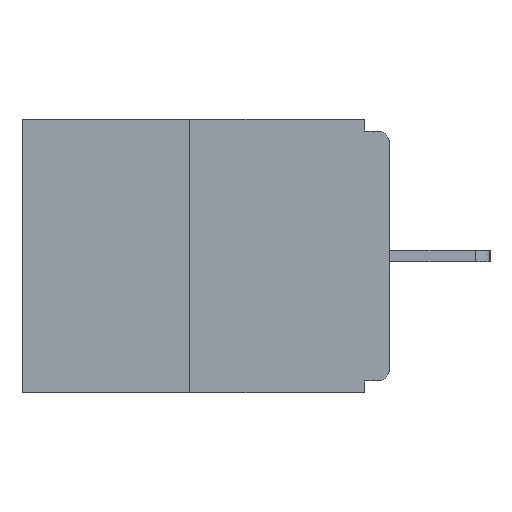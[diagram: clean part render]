
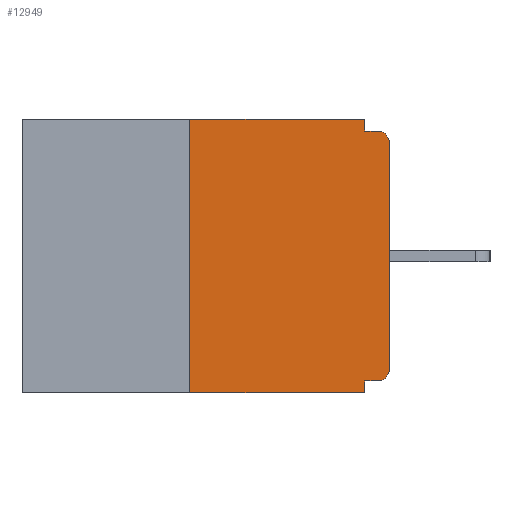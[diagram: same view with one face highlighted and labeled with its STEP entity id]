
A CAD part, left-side view. The second image highlights one B-rep face of the part: STEP entity #12949.
In plain terms, the highlighted planar face has unit normal (-1, 0, 0).
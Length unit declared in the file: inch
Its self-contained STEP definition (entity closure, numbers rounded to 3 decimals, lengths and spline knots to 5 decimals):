
#451 = ORIENTED_EDGE ( 'NONE', *, *, #3247, .T. ) ;
#538 = VERTEX_POINT ( 'NONE', #2615 ) ;
#864 = EDGE_CURVE ( 'NONE', #14884, #14288, #8398, .T. ) ;
#1277 = DIRECTION ( 'NONE',  ( 0., -1., 0. ) ) ;
#1319 = EDGE_CURVE ( 'NONE', #538, #14288, #9498, .T. ) ;
#2554 = PLANE ( 'NONE',  #6915 ) ;
#2615 = CARTESIAN_POINT ( 'NONE',  ( 0., 0.031, -0.015 ) ) ;
#2713 = EDGE_CURVE ( 'NONE', #12094, #3547, #5743, .T. ) ;
#3247 = EDGE_CURVE ( 'NONE', #9905, #14884, #15574, .T. ) ;
#3251 = VERTEX_POINT ( 'NONE', #15971 ) ;
#3293 = CARTESIAN_POINT ( 'NONE',  ( 0., 0.031, 0. ) ) ;
#3547 = VERTEX_POINT ( 'NONE', #12677 ) ;
#3567 = ORIENTED_EDGE ( 'NONE', *, *, #11888, .F. ) ;
#3789 = FACE_OUTER_BOUND ( 'NONE', #4753, .T. ) ;
#4266 = ORIENTED_EDGE ( 'NONE', *, *, #2713, .F. ) ;
#4335 = DIRECTION ( 'NONE',  ( 0., 0., 1. ) ) ;
#4632 = DIRECTION ( 'NONE',  ( 0., -1., 0. ) ) ;
#4753 = EDGE_LOOP ( 'NONE', ( #9517, #4266, #13610, #5436, #12187, #16011, #451, #15184, #11921, #3567 ) ) ;
#4779 = DIRECTION ( 'NONE',  ( 0., 1., 0. ) ) ;
#5211 = CARTESIAN_POINT ( 'NONE',  ( 0., 0.015, -0.328 ) ) ;
#5270 = VECTOR ( 'NONE', #14427, 39.37008 ) ;
#5340 = LINE ( 'NONE', #10348, #9208 ) ;
#5436 = ORIENTED_EDGE ( 'NONE', *, *, #7904, .F. ) ;
#5743 = LINE ( 'NONE', #9524, #14557 ) ;
#6101 = AXIS2_PLACEMENT_3D ( 'NONE', #10490, #6330, #6714 ) ;
#6148 = LINE ( 'NONE', #16160, #8930 ) ;
#6330 = DIRECTION ( 'NONE',  ( -1., 0., 0. ) ) ;
#6335 = DIRECTION ( 'NONE',  ( 0., 0., -1. ) ) ;
#6344 = EDGE_CURVE ( 'NONE', #3547, #9512, #6148, .T. ) ;
#6607 = VECTOR ( 'NONE', #4779, 39.37008 ) ;
#6714 = DIRECTION ( 'NONE',  ( 0., 0., -1. ) ) ;
#6915 = AXIS2_PLACEMENT_3D ( 'NONE', #12328, #7566, #6335 ) ;
#7176 = LINE ( 'NONE', #8628, #6607 ) ;
#7566 = DIRECTION ( 'NONE',  ( 1., 0., 0. ) ) ;
#7615 = AXIS2_PLACEMENT_3D ( 'NONE', #15914, #12053, #13526 ) ;
#7760 = EDGE_CURVE ( 'NONE', #8269, #9905, #13180, .T. ) ;
#7904 = EDGE_CURVE ( 'NONE', #3251, #12931, #8270, .T. ) ;
#8196 = CARTESIAN_POINT ( 'NONE',  ( 0., 0.031, -0.343 ) ) ;
#8269 = VERTEX_POINT ( 'NONE', #5211 ) ;
#8270 = LINE ( 'NONE', #8196, #5270 ) ;
#8398 = CIRCLE ( 'NONE', #7615, 0.015 ) ;
#8628 = CARTESIAN_POINT ( 'NONE',  ( 0., 0., -0.328 ) ) ;
#8690 = CARTESIAN_POINT ( 'NONE',  ( 0., 0.25, -0.343 ) ) ;
#8851 = EDGE_CURVE ( 'NONE', #8269, #3251, #7176, .T. ) ;
#8930 = VECTOR ( 'NONE', #1277, 39.37008 ) ;
#9208 = VECTOR ( 'NONE', #15346, 39.37008 ) ;
#9333 = DIRECTION ( 'NONE',  ( 0., 0., 1. ) ) ;
#9445 = DIRECTION ( 'NONE',  ( 0., 0., -1. ) ) ;
#9498 = LINE ( 'NONE', #15888, #11288 ) ;
#9512 = VERTEX_POINT ( 'NONE', #13851 ) ;
#9517 = ORIENTED_EDGE ( 'NONE', *, *, #6344, .F. ) ;
#9524 = CARTESIAN_POINT ( 'NONE',  ( 0., 0.25, 0. ) ) ;
#9643 = VECTOR ( 'NONE', #9333, 39.37008 ) ;
#9905 = VERTEX_POINT ( 'NONE', #12747 ) ;
#9947 = CARTESIAN_POINT ( 'NONE',  ( 0., 0., -0.03 ) ) ;
#10348 = CARTESIAN_POINT ( 'NONE',  ( 0., 0.46, -0.343 ) ) ;
#10490 = CARTESIAN_POINT ( 'NONE',  ( 0., 0.015, -0.313 ) ) ;
#10599 = EDGE_CURVE ( 'NONE', #12094, #12931, #5340, .T. ) ;
#11288 = VECTOR ( 'NONE', #4632, 39.37008 ) ;
#11347 = CARTESIAN_POINT ( 'NONE',  ( 0., 0.031, -0.343 ) ) ;
#11888 = EDGE_CURVE ( 'NONE', #9512, #538, #13299, .T. ) ;
#11921 = ORIENTED_EDGE ( 'NONE', *, *, #1319, .F. ) ;
#12053 = DIRECTION ( 'NONE',  ( -1., 0., 0. ) ) ;
#12094 = VERTEX_POINT ( 'NONE', #8690 ) ;
#12187 = ORIENTED_EDGE ( 'NONE', *, *, #8851, .F. ) ;
#12328 = CARTESIAN_POINT ( 'NONE',  ( 0., 0.46, 0. ) ) ;
#12677 = CARTESIAN_POINT ( 'NONE',  ( 0., 0.25, 0. ) ) ;
#12747 = CARTESIAN_POINT ( 'NONE',  ( 0., 0., -0.313 ) ) ;
#12931 = VERTEX_POINT ( 'NONE', #11347 ) ;
#12949 = ADVANCED_FACE ( 'NONE', ( #3789 ), #2554, .F. ) ;
#13180 = CIRCLE ( 'NONE', #6101, 0.015 ) ;
#13299 = LINE ( 'NONE', #3293, #13695 ) ;
#13526 = DIRECTION ( 'NONE',  ( 0., 0., -1. ) ) ;
#13610 = ORIENTED_EDGE ( 'NONE', *, *, #10599, .T. ) ;
#13695 = VECTOR ( 'NONE', #9445, 39.37008 ) ;
#13851 = CARTESIAN_POINT ( 'NONE',  ( 0., 0.031, 0. ) ) ;
#14288 = VERTEX_POINT ( 'NONE', #15884 ) ;
#14417 = CARTESIAN_POINT ( 'NONE',  ( 0., 0., 0. ) ) ;
#14427 = DIRECTION ( 'NONE',  ( 0., 0., -1. ) ) ;
#14557 = VECTOR ( 'NONE', #4335, 39.37008 ) ;
#14884 = VERTEX_POINT ( 'NONE', #9947 ) ;
#15184 = ORIENTED_EDGE ( 'NONE', *, *, #864, .T. ) ;
#15346 = DIRECTION ( 'NONE',  ( 0., -1., 0. ) ) ;
#15574 = LINE ( 'NONE', #14417, #9643 ) ;
#15884 = CARTESIAN_POINT ( 'NONE',  ( 0., 0.015, -0.015 ) ) ;
#15888 = CARTESIAN_POINT ( 'NONE',  ( 0., 0., -0.015 ) ) ;
#15914 = CARTESIAN_POINT ( 'NONE',  ( 0., 0.015, -0.03 ) ) ;
#15971 = CARTESIAN_POINT ( 'NONE',  ( 0., 0.031, -0.328 ) ) ;
#16011 = ORIENTED_EDGE ( 'NONE', *, *, #7760, .T. ) ;
#16160 = CARTESIAN_POINT ( 'NONE',  ( 0., 0.46, 0. ) ) ;
